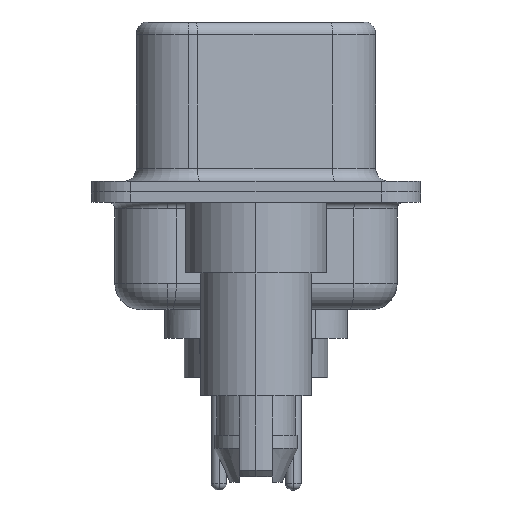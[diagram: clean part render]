
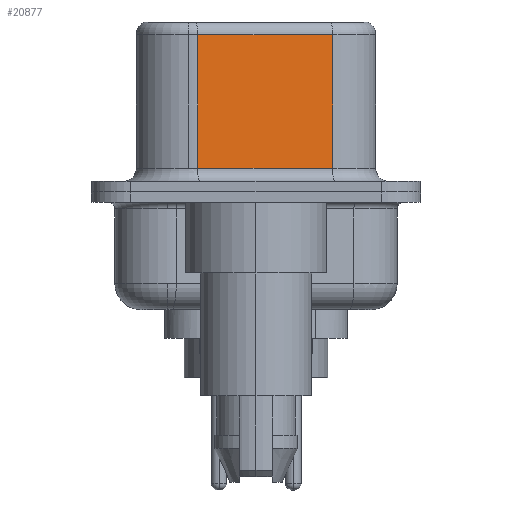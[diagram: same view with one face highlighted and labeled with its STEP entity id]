
A CAD part, left-side view. The second image highlights one B-rep face of the part: STEP entity #20877.
In plain terms, the highlighted planar face has unit normal (-0.985, -0.174, 0).
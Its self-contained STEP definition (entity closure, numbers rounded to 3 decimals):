
#757 = DIRECTION ( 'NONE',  ( -0.174, 0.985, 0. ) ) ;
#1270 = DIRECTION ( 'NONE',  ( 0., 0., -1. ) ) ;
#1645 = VECTOR ( 'NONE', #14178, 1000. ) ;
#3452 = CARTESIAN_POINT ( 'NONE',  ( 3.655, 2.233, 0.9 ) ) ;
#3849 = LINE ( 'NONE', #18362, #7759 ) ;
#3925 = EDGE_CURVE ( 'NONE', #9983, #13916, #3849, .T. ) ;
#3975 = AXIS2_PLACEMENT_3D ( 'NONE', #8532, #17190, #6853 ) ;
#4921 = EDGE_CURVE ( 'NONE', #9585, #11482, #18542, .T. ) ;
#5181 = PLANE ( 'NONE',  #3975 ) ;
#5378 = VECTOR ( 'NONE', #1270, 1000. ) ;
#6853 = DIRECTION ( 'NONE',  ( -0.174, 0.985, 0. ) ) ;
#7197 = LINE ( 'NONE', #17680, #1645 ) ;
#7309 = CARTESIAN_POINT ( 'NONE',  ( 4.565, -2.927, 0.9 ) ) ;
#7759 = VECTOR ( 'NONE', #19295, 1000. ) ;
#8532 = CARTESIAN_POINT ( 'NONE',  ( 4.565, -2.927, 6.52 ) ) ;
#9585 = VERTEX_POINT ( 'NONE', #15109 ) ;
#9983 = VERTEX_POINT ( 'NONE', #12927 ) ;
#10850 = ORIENTED_EDGE ( 'NONE', *, *, #3925, .T. ) ;
#10969 = VECTOR ( 'NONE', #757, 1000. ) ;
#11167 = ORIENTED_EDGE ( 'NONE', *, *, #21306, .T. ) ;
#11482 = VERTEX_POINT ( 'NONE', #7309 ) ;
#12154 = CARTESIAN_POINT ( 'NONE',  ( 4.565, -2.927, 6.52 ) ) ;
#12819 = CARTESIAN_POINT ( 'NONE',  ( 4.565, -2.927, 6.02 ) ) ;
#12927 = CARTESIAN_POINT ( 'NONE',  ( 3.655, 2.233, 6.02 ) ) ;
#13758 = ORIENTED_EDGE ( 'NONE', *, *, #18427, .T. ) ;
#13916 = VERTEX_POINT ( 'NONE', #3452 ) ;
#14178 = DIRECTION ( 'NONE',  ( 0.174, -0.985, 0. ) ) ;
#14673 = ORIENTED_EDGE ( 'NONE', *, *, #4921, .F. ) ;
#15028 = LINE ( 'NONE', #12819, #10969 ) ;
#15109 = CARTESIAN_POINT ( 'NONE',  ( 4.565, -2.927, 6.02 ) ) ;
#15295 = FACE_OUTER_BOUND ( 'NONE', #18530, .T. ) ;
#17190 = DIRECTION ( 'NONE',  ( 0.985, 0.174, 0. ) ) ;
#17680 = CARTESIAN_POINT ( 'NONE',  ( 4.565, -2.927, 0.9 ) ) ;
#18362 = CARTESIAN_POINT ( 'NONE',  ( 3.655, 2.233, 6.52 ) ) ;
#18427 = EDGE_CURVE ( 'NONE', #13916, #11482, #7197, .T. ) ;
#18530 = EDGE_LOOP ( 'NONE', ( #14673, #11167, #10850, #13758 ) ) ;
#18542 = LINE ( 'NONE', #12154, #5378 ) ;
#19295 = DIRECTION ( 'NONE',  ( 0., 0., -1. ) ) ;
#20877 = ADVANCED_FACE ( 'NONE', ( #15295 ), #5181, .F. ) ;
#21306 = EDGE_CURVE ( 'NONE', #9585, #9983, #15028, .T. ) ;
